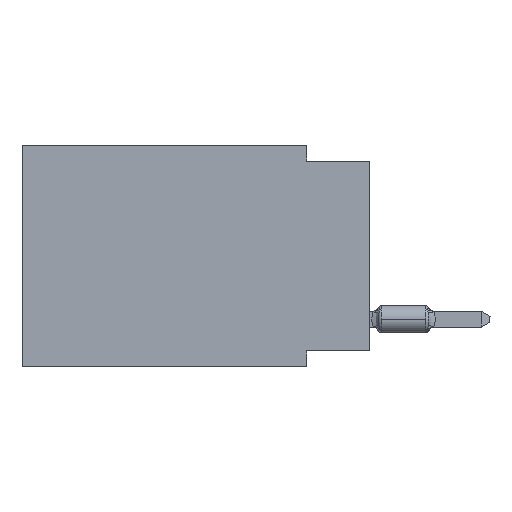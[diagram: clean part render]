
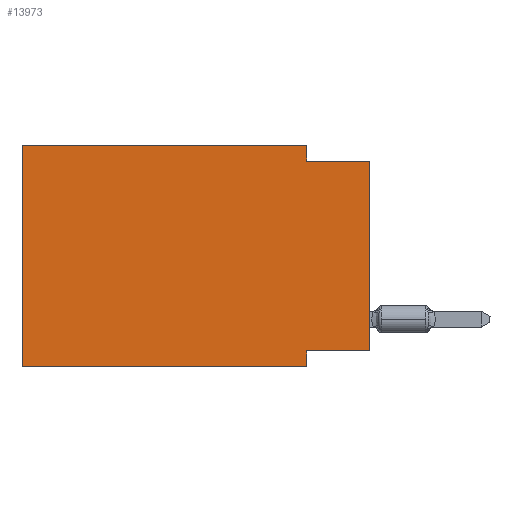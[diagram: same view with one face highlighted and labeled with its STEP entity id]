
A CAD part, left-side view. The second image highlights one B-rep face of the part: STEP entity #13973.
In plain terms, the highlighted planar face has unit normal (-1, 0, 0).
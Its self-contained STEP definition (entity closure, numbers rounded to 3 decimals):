
#1868 = AXIS2_PLACEMENT_3D ( 'NONE', #13155, #36404, #59647 ) ;
#7850 = VECTOR ( 'NONE', #26676, 1000. ) ;
#9530 = DIRECTION ( 'NONE',  ( 0., 1., 0. ) ) ;
#9924 = DIRECTION ( 'NONE',  ( 0., 0., 1. ) ) ;
#10250 = LINE ( 'NONE', #16354, #28992 ) ;
#10396 = LINE ( 'NONE', #51544, #30981 ) ;
#13155 = CARTESIAN_POINT ( 'NONE',  ( 0., 13.97, 0. ) ) ;
#13973 = ADVANCED_FACE ( 'NONE', ( #58123 ), #30307, .F. ) ;
#16354 = CARTESIAN_POINT ( 'NONE',  ( 0., 0., -0.635 ) ) ;
#16692 = ORIENTED_EDGE ( 'NONE', *, *, #28730, .F. ) ;
#17023 = VERTEX_POINT ( 'NONE', #38330 ) ;
#18970 = EDGE_CURVE ( 'NONE', #51498, #61349, #74323, .T. ) ;
#21341 = LINE ( 'NONE', #56763, #32235 ) ;
#24341 = EDGE_LOOP ( 'NONE', ( #58449, #65209, #75208, #45954, #27217, #59858, #16692, #52022 ) ) ;
#24538 = VECTOR ( 'NONE', #36100, 1000. ) ;
#25040 = EDGE_CURVE ( 'NONE', #51498, #17023, #21341, .T. ) ;
#25306 = VECTOR ( 'NONE', #65644, 1000. ) ;
#26676 = DIRECTION ( 'NONE',  ( 0., 0., -1. ) ) ;
#27198 = VERTEX_POINT ( 'NONE', #72436 ) ;
#27217 = ORIENTED_EDGE ( 'NONE', *, *, #52680, .F. ) ;
#27692 = CARTESIAN_POINT ( 'NONE',  ( 0., 13.97, 0. ) ) ;
#27849 = VECTOR ( 'NONE', #53873, 1000. ) ;
#28730 = EDGE_CURVE ( 'NONE', #17023, #38200, #44207, .T. ) ;
#28992 = VECTOR ( 'NONE', #34258, 1000. ) ;
#30307 = PLANE ( 'NONE',  #1868 ) ;
#30391 = CARTESIAN_POINT ( 'NONE',  ( 0., 13.97, 0. ) ) ;
#30649 = CARTESIAN_POINT ( 'NONE',  ( 0., 13.97, -8.89 ) ) ;
#30981 = VECTOR ( 'NONE', #74802, 1000. ) ;
#32235 = VECTOR ( 'NONE', #9530, 1000. ) ;
#34258 = DIRECTION ( 'NONE',  ( 0., -1., 0. ) ) ;
#34374 = EDGE_CURVE ( 'NONE', #40518, #58345, #36686, .T. ) ;
#35426 = CARTESIAN_POINT ( 'NONE',  ( 0., 2.54, -8.89 ) ) ;
#36100 = DIRECTION ( 'NONE',  ( 0., 0., 1. ) ) ;
#36404 = DIRECTION ( 'NONE',  ( 1., 0., 0. ) ) ;
#36686 = LINE ( 'NONE', #37040, #25306 ) ;
#37040 = CARTESIAN_POINT ( 'NONE',  ( 0., 13.97, 0. ) ) ;
#37105 = LINE ( 'NONE', #30649, #27849 ) ;
#37893 = LINE ( 'NONE', #30391, #24538 ) ;
#38200 = VERTEX_POINT ( 'NONE', #35426 ) ;
#38330 = CARTESIAN_POINT ( 'NONE',  ( 0., 2.54, -8.255 ) ) ;
#40518 = VERTEX_POINT ( 'NONE', #27692 ) ;
#43858 = CARTESIAN_POINT ( 'NONE',  ( 0., 2.54, -0.635 ) ) ;
#44207 = LINE ( 'NONE', #55625, #7850 ) ;
#44321 = CARTESIAN_POINT ( 'NONE',  ( 0., 0., -8.255 ) ) ;
#45570 = CARTESIAN_POINT ( 'NONE',  ( 0., 0., -0.635 ) ) ;
#45954 = ORIENTED_EDGE ( 'NONE', *, *, #34374, .F. ) ;
#51498 = VERTEX_POINT ( 'NONE', #44321 ) ;
#51544 = CARTESIAN_POINT ( 'NONE',  ( 0., 2.54, 0. ) ) ;
#52022 = ORIENTED_EDGE ( 'NONE', *, *, #25040, .F. ) ;
#52680 = EDGE_CURVE ( 'NONE', #27198, #40518, #37893, .T. ) ;
#53873 = DIRECTION ( 'NONE',  ( 0., -1., 0. ) ) ;
#55625 = CARTESIAN_POINT ( 'NONE',  ( 0., 2.54, -8.89 ) ) ;
#56763 = CARTESIAN_POINT ( 'NONE',  ( 0., 0., -8.255 ) ) ;
#58123 = FACE_OUTER_BOUND ( 'NONE', #24341, .T. ) ;
#58345 = VERTEX_POINT ( 'NONE', #73606 ) ;
#58449 = ORIENTED_EDGE ( 'NONE', *, *, #18970, .T. ) ;
#59647 = DIRECTION ( 'NONE',  ( 0., 0., -1. ) ) ;
#59858 = ORIENTED_EDGE ( 'NONE', *, *, #73199, .T. ) ;
#61349 = VERTEX_POINT ( 'NONE', #45570 ) ;
#65209 = ORIENTED_EDGE ( 'NONE', *, *, #72664, .F. ) ;
#65644 = DIRECTION ( 'NONE',  ( 0., -1., 0. ) ) ;
#66283 = VERTEX_POINT ( 'NONE', #43858 ) ;
#67186 = EDGE_CURVE ( 'NONE', #58345, #66283, #10396, .T. ) ;
#72436 = CARTESIAN_POINT ( 'NONE',  ( 0., 13.97, -8.89 ) ) ;
#72664 = EDGE_CURVE ( 'NONE', #66283, #61349, #10250, .T. ) ;
#73028 = VECTOR ( 'NONE', #9924, 1000. ) ;
#73199 = EDGE_CURVE ( 'NONE', #27198, #38200, #37105, .T. ) ;
#73606 = CARTESIAN_POINT ( 'NONE',  ( 0., 2.54, 0. ) ) ;
#74323 = LINE ( 'NONE', #75060, #73028 ) ;
#74802 = DIRECTION ( 'NONE',  ( 0., 0., -1. ) ) ;
#75060 = CARTESIAN_POINT ( 'NONE',  ( 0., 0., 0. ) ) ;
#75208 = ORIENTED_EDGE ( 'NONE', *, *, #67186, .F. ) ;
